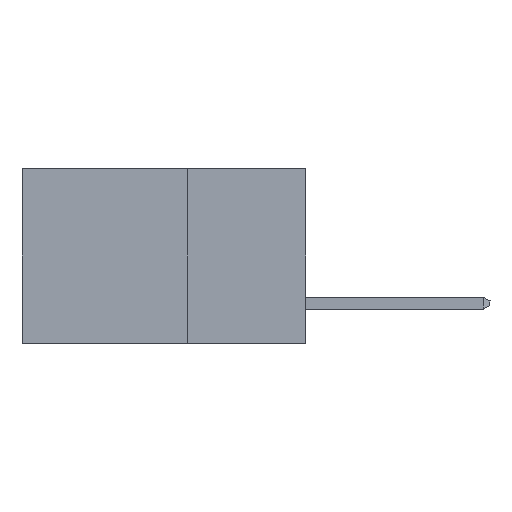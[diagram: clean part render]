
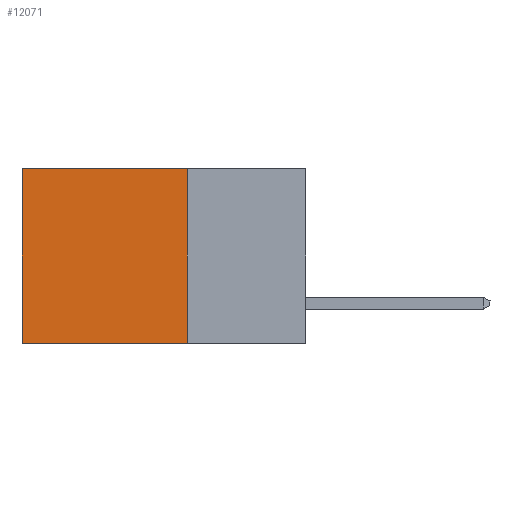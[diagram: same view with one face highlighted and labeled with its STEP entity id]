
A CAD part, left-side view. The second image highlights one B-rep face of the part: STEP entity #12071.
In plain terms, the highlighted planar face has unit normal (-1, 0, 0).
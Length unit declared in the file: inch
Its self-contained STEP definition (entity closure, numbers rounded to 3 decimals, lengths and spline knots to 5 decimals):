
#29 = DIRECTION ( 'NONE',  ( 0., 1., 0. ) ) ;
#247 = EDGE_CURVE ( 'NONE', #11538, #10820, #7595, .T. ) ;
#635 = CARTESIAN_POINT ( 'NONE',  ( 0.298, 0.25, 0. ) ) ;
#669 = EDGE_CURVE ( 'NONE', #11538, #13439, #12016, .T. ) ;
#1328 = DIRECTION ( 'NONE',  ( 0., 0., -1. ) ) ;
#1987 = VECTOR ( 'NONE', #10410, 39.37008 ) ;
#2073 = ORIENTED_EDGE ( 'NONE', *, *, #13181, .T. ) ;
#2189 = DIRECTION ( 'NONE',  ( 0., 1., 0. ) ) ;
#2406 = EDGE_CURVE ( 'NONE', #13439, #3462, #6425, .T. ) ;
#2458 = AXIS2_PLACEMENT_3D ( 'NONE', #13032, #3725, #1328 ) ;
#2753 = ORIENTED_EDGE ( 'NONE', *, *, #2406, .F. ) ;
#3462 = VERTEX_POINT ( 'NONE', #8821 ) ;
#3725 = DIRECTION ( 'NONE',  ( 1., 0., 0. ) ) ;
#4185 = DIRECTION ( 'NONE',  ( 0., 0., -1. ) ) ;
#4693 = CARTESIAN_POINT ( 'NONE',  ( 0.298, 0.25, 0. ) ) ;
#5019 = FACE_OUTER_BOUND ( 'NONE', #8288, .T. ) ;
#5058 = ORIENTED_EDGE ( 'NONE', *, *, #247, .T. ) ;
#5947 = CARTESIAN_POINT ( 'NONE',  ( 0.298, 0.6, 0. ) ) ;
#6425 = LINE ( 'NONE', #11791, #14190 ) ;
#6755 = LINE ( 'NONE', #5947, #1987 ) ;
#7595 = LINE ( 'NONE', #635, #9597 ) ;
#8288 = EDGE_LOOP ( 'NONE', ( #2073, #2753, #12382, #5058 ) ) ;
#8821 = CARTESIAN_POINT ( 'NONE',  ( 0.298, 0.6, -0.37 ) ) ;
#9597 = VECTOR ( 'NONE', #2189, 39.37008 ) ;
#9873 = CARTESIAN_POINT ( 'NONE',  ( 0.298, 0.25, 0. ) ) ;
#10410 = DIRECTION ( 'NONE',  ( 0., 0., -1. ) ) ;
#10820 = VERTEX_POINT ( 'NONE', #11524 ) ;
#11524 = CARTESIAN_POINT ( 'NONE',  ( 0.298, 0.6, 0. ) ) ;
#11538 = VERTEX_POINT ( 'NONE', #4693 ) ;
#11791 = CARTESIAN_POINT ( 'NONE',  ( 0.298, 0.25, -0.37 ) ) ;
#12016 = LINE ( 'NONE', #9873, #12553 ) ;
#12071 = ADVANCED_FACE ( 'NONE', ( #5019 ), #13085, .F. ) ;
#12122 = CARTESIAN_POINT ( 'NONE',  ( 0.298, 0.25, -0.37 ) ) ;
#12382 = ORIENTED_EDGE ( 'NONE', *, *, #669, .F. ) ;
#12553 = VECTOR ( 'NONE', #4185, 39.37008 ) ;
#13032 = CARTESIAN_POINT ( 'NONE',  ( 0.298, 0.25, 0. ) ) ;
#13085 = PLANE ( 'NONE',  #2458 ) ;
#13181 = EDGE_CURVE ( 'NONE', #10820, #3462, #6755, .T. ) ;
#13439 = VERTEX_POINT ( 'NONE', #12122 ) ;
#14190 = VECTOR ( 'NONE', #29, 39.37008 ) ;
